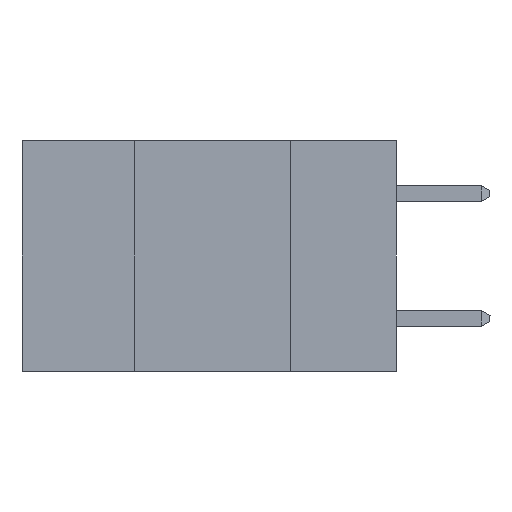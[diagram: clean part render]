
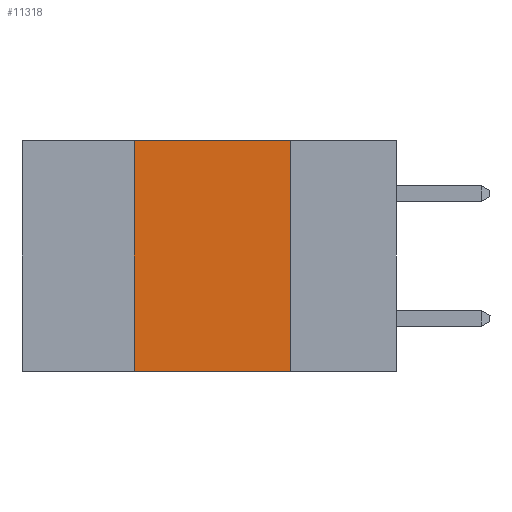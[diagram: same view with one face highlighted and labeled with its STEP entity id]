
A CAD part, left-side view. The second image highlights one B-rep face of the part: STEP entity #11318.
In plain terms, the highlighted planar face has unit normal (-1, 0, 0).
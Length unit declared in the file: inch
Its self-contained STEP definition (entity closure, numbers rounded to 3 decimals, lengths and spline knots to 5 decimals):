
#179 = DIRECTION ( 'NONE',  ( 0., 0., -1. ) ) ;
#939 = LINE ( 'NONE', #18571, #16728 ) ;
#1341 = LINE ( 'NONE', #9578, #16653 ) ;
#1958 = DIRECTION ( 'NONE',  ( 0., -1., 0. ) ) ;
#2213 = VERTEX_POINT ( 'NONE', #14553 ) ;
#2279 = LINE ( 'NONE', #14906, #5919 ) ;
#2332 = DIRECTION ( 'NONE',  ( 0., 0., -1. ) ) ;
#2825 = ORIENTED_EDGE ( 'NONE', *, *, #14043, .F. ) ;
#2945 = ORIENTED_EDGE ( 'NONE', *, *, #3239, .T. ) ;
#3239 = EDGE_CURVE ( 'NONE', #15109, #2213, #2279, .T. ) ;
#3443 = CARTESIAN_POINT ( 'NONE',  ( 0., 0.17, 0. ) ) ;
#4257 = VECTOR ( 'NONE', #2332, 39.37008 ) ;
#4752 = LINE ( 'NONE', #12808, #4257 ) ;
#5919 = VECTOR ( 'NONE', #14470, 39.37008 ) ;
#6332 = PLANE ( 'NONE',  #9976 ) ;
#7269 = FACE_OUTER_BOUND ( 'NONE', #10332, .T. ) ;
#7487 = CARTESIAN_POINT ( 'NONE',  ( 0., 0.42, 0. ) ) ;
#9347 = DIRECTION ( 'NONE',  ( 1., 0., 0. ) ) ;
#9578 = CARTESIAN_POINT ( 'NONE',  ( 0., 0.6, 0. ) ) ;
#9976 = AXIS2_PLACEMENT_3D ( 'NONE', #16496, #9347, #179 ) ;
#10332 = EDGE_LOOP ( 'NONE', ( #2825, #11127, #15208, #2945 ) ) ;
#11127 = ORIENTED_EDGE ( 'NONE', *, *, #15099, .F. ) ;
#11318 = ADVANCED_FACE ( 'NONE', ( #7269 ), #6332, .F. ) ;
#11442 = DIRECTION ( 'NONE',  ( 0., 0., 1. ) ) ;
#12808 = CARTESIAN_POINT ( 'NONE',  ( 0., 0.17, -0.37 ) ) ;
#13400 = EDGE_CURVE ( 'NONE', #15109, #13620, #939, .T. ) ;
#13620 = VERTEX_POINT ( 'NONE', #7487 ) ;
#14043 = EDGE_CURVE ( 'NONE', #18691, #2213, #4752, .T. ) ;
#14470 = DIRECTION ( 'NONE',  ( 0., -1., 0. ) ) ;
#14553 = CARTESIAN_POINT ( 'NONE',  ( 0., 0.17, -0.37 ) ) ;
#14906 = CARTESIAN_POINT ( 'NONE',  ( 0., 0.6, -0.37 ) ) ;
#15099 = EDGE_CURVE ( 'NONE', #13620, #18691, #1341, .T. ) ;
#15109 = VERTEX_POINT ( 'NONE', #15330 ) ;
#15208 = ORIENTED_EDGE ( 'NONE', *, *, #13400, .F. ) ;
#15330 = CARTESIAN_POINT ( 'NONE',  ( 0., 0.42, -0.37 ) ) ;
#16496 = CARTESIAN_POINT ( 'NONE',  ( 0., 0.6, 0. ) ) ;
#16653 = VECTOR ( 'NONE', #1958, 39.37008 ) ;
#16728 = VECTOR ( 'NONE', #11442, 39.37008 ) ;
#18571 = CARTESIAN_POINT ( 'NONE',  ( 0., 0.42, -0.37 ) ) ;
#18691 = VERTEX_POINT ( 'NONE', #3443 ) ;
